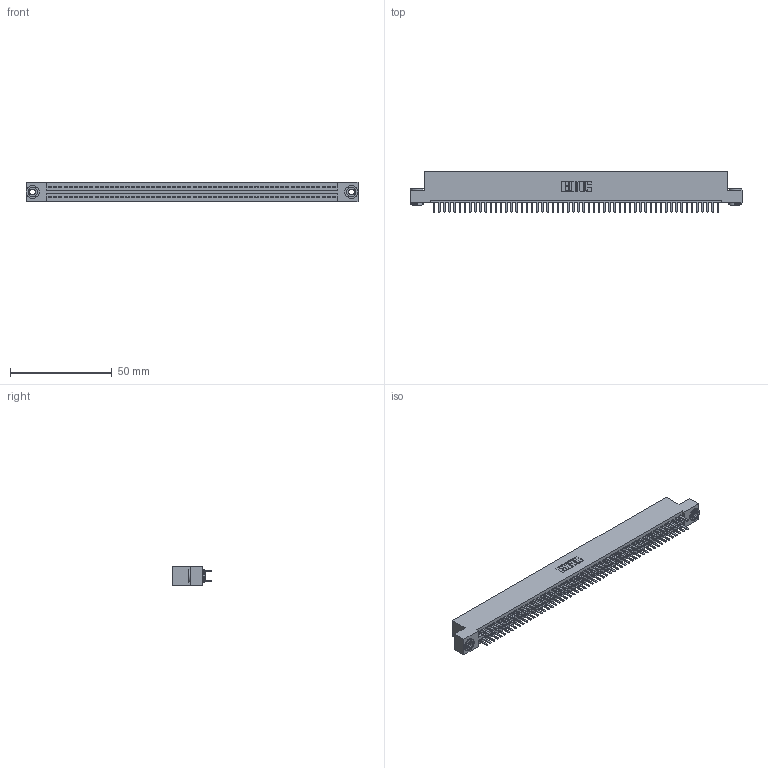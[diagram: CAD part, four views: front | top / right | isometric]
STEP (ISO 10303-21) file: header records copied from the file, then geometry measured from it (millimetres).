
FILE_DESCRIPTION (( 'STEP AP203' ), '1' );
FILE_NAME ('395-112-520-203.STEP', '2018-12-01T06:51:43', ( '' ), ( '' ), 'SwSTEP 2.0', 'SolidWorks 2016', '' );
FILE_SCHEMA (( 'CONFIG_CONTROL_DESIGN' ));
Length unit declared in the file: inch
Products named in the file (4): 345 Part_Flush Mounting Lugs - 0.156 Dia-TH; 395-112-520-203; 345-292-001_345-293-120; 345-250-002_345-250-002-102
Assembly tree (115 placements, depth 2):
  395-112-520-203
    345 Part_Flush Mounting Lugs - 0.156 Dia-TH
    345-292-001_345-293-120  x112
    345-250-002_345-250-002-102  x2
Bounding box: 163.45 x 19.68 x 9.4 mm (x, y, z)
Volume: 15977.7 mm3; surface area: 23989.1 mm2
Topology: 115 solids, 115 shells, 6212 faces, 18001 edges, 11698 vertices
Faces by surface type: plane 4010, cylinder 2194, cone 8
Entity records: 42818 total; most frequent: CARTESIAN_POINT 7151, ORIENTED_EDGE 7066, DIRECTION 6307, EDGE_CURVE 3533, VECTOR 3149, LINE 3149, VERTEX_POINT 2350, AXIS2_PLACEMENT_3D 1579
